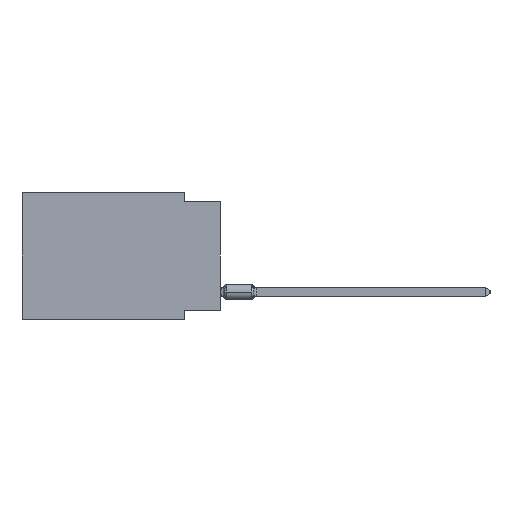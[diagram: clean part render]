
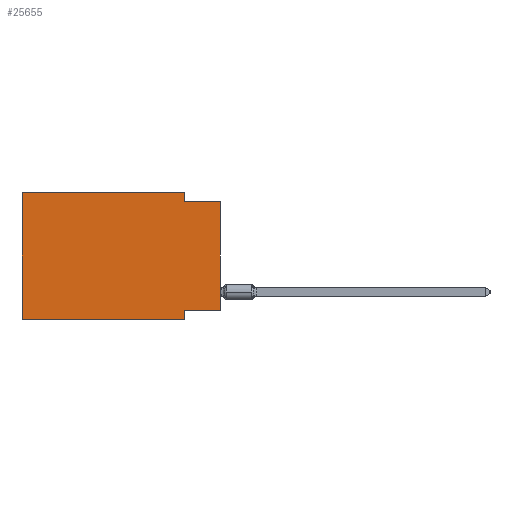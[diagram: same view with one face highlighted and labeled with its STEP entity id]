
A CAD part, left-side view. The second image highlights one B-rep face of the part: STEP entity #25655.
In plain terms, the highlighted planar face has unit normal (-1, 0, 0).
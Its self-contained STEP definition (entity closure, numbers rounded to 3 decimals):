
#2280 = VECTOR ( 'NONE', #48799, 1000. ) ;
#2856 = DIRECTION ( 'NONE',  ( 0., 1., 0. ) ) ;
#3340 = LINE ( 'NONE', #44732, #25423 ) ;
#3586 = CARTESIAN_POINT ( 'NONE',  ( 0., 13.97, 0. ) ) ;
#4630 = EDGE_LOOP ( 'NONE', ( #45822, #41184, #35078, #54529, #61562, #39311, #8893, #6857 ) ) ;
#4835 = EDGE_CURVE ( 'NONE', #22726, #38646, #18405, .T. ) ;
#6857 = ORIENTED_EDGE ( 'NONE', *, *, #37239, .F. ) ;
#8236 = CARTESIAN_POINT ( 'NONE',  ( 0., 2.54, -8.89 ) ) ;
#8479 = VECTOR ( 'NONE', #18309, 1000. ) ;
#8893 = ORIENTED_EDGE ( 'NONE', *, *, #59801, .F. ) ;
#9048 = PLANE ( 'NONE',  #47909 ) ;
#10798 = LINE ( 'NONE', #46864, #11913 ) ;
#11913 = VECTOR ( 'NONE', #29905, 1000. ) ;
#12756 = VERTEX_POINT ( 'NONE', #59773 ) ;
#14596 = CARTESIAN_POINT ( 'NONE',  ( 0., 2.54, 0. ) ) ;
#17453 = CARTESIAN_POINT ( 'NONE',  ( 0., 13.97, 0. ) ) ;
#18309 = DIRECTION ( 'NONE',  ( 0., -1., 0. ) ) ;
#18405 = LINE ( 'NONE', #28412, #2280 ) ;
#18553 = CARTESIAN_POINT ( 'NONE',  ( 0., 13.97, -8.89 ) ) ;
#19028 = VERTEX_POINT ( 'NONE', #32511 ) ;
#19071 = VERTEX_POINT ( 'NONE', #37526 ) ;
#19079 = DIRECTION ( 'NONE',  ( 1., 0., 0. ) ) ;
#19621 = LINE ( 'NONE', #28971, #8479 ) ;
#22726 = VERTEX_POINT ( 'NONE', #17453 ) ;
#24080 = VERTEX_POINT ( 'NONE', #52209 ) ;
#24137 = CARTESIAN_POINT ( 'NONE',  ( 0., 2.54, -8.255 ) ) ;
#24766 = VERTEX_POINT ( 'NONE', #59408 ) ;
#25423 = VECTOR ( 'NONE', #39058, 1000. ) ;
#25655 = ADVANCED_FACE ( 'NONE', ( #39110 ), #9048, .F. ) ;
#28234 = LINE ( 'NONE', #48616, #57501 ) ;
#28412 = CARTESIAN_POINT ( 'NONE',  ( 0., 13.97, 0. ) ) ;
#28971 = CARTESIAN_POINT ( 'NONE',  ( 0., 0., -0.635 ) ) ;
#29158 = EDGE_CURVE ( 'NONE', #19028, #24080, #10798, .T. ) ;
#29258 = DIRECTION ( 'NONE',  ( 0., 0., -1. ) ) ;
#29408 = CARTESIAN_POINT ( 'NONE',  ( 0., 13.97, 0. ) ) ;
#29905 = DIRECTION ( 'NONE',  ( 0., 0., 1. ) ) ;
#32064 = VERTEX_POINT ( 'NONE', #24137 ) ;
#32511 = CARTESIAN_POINT ( 'NONE',  ( 0., 0., -8.255 ) ) ;
#34122 = DIRECTION ( 'NONE',  ( 0., 0., -1. ) ) ;
#35078 = ORIENTED_EDGE ( 'NONE', *, *, #47516, .F. ) ;
#37239 = EDGE_CURVE ( 'NONE', #19028, #32064, #28234, .T. ) ;
#37526 = CARTESIAN_POINT ( 'NONE',  ( 0., 13.97, -8.89 ) ) ;
#38620 = EDGE_CURVE ( 'NONE', #24766, #24080, #19621, .T. ) ;
#38646 = VERTEX_POINT ( 'NONE', #14596 ) ;
#38920 = EDGE_CURVE ( 'NONE', #19071, #12756, #54632, .T. ) ;
#39058 = DIRECTION ( 'NONE',  ( 0., 0., -1. ) ) ;
#39110 = FACE_OUTER_BOUND ( 'NONE', #4630, .T. ) ;
#39311 = ORIENTED_EDGE ( 'NONE', *, *, #38920, .T. ) ;
#39898 = DIRECTION ( 'NONE',  ( 0., -1., 0. ) ) ;
#41184 = ORIENTED_EDGE ( 'NONE', *, *, #38620, .F. ) ;
#44732 = CARTESIAN_POINT ( 'NONE',  ( 0., 2.54, 0. ) ) ;
#45822 = ORIENTED_EDGE ( 'NONE', *, *, #29158, .T. ) ;
#46844 = VECTOR ( 'NONE', #29258, 1000. ) ;
#46864 = CARTESIAN_POINT ( 'NONE',  ( 0., 0., 0. ) ) ;
#47516 = EDGE_CURVE ( 'NONE', #38646, #24766, #3340, .T. ) ;
#47909 = AXIS2_PLACEMENT_3D ( 'NONE', #29408, #19079, #34122 ) ;
#48104 = VECTOR ( 'NONE', #50328, 1000. ) ;
#48616 = CARTESIAN_POINT ( 'NONE',  ( 0., 0., -8.255 ) ) ;
#48799 = DIRECTION ( 'NONE',  ( 0., -1., 0. ) ) ;
#49345 = LINE ( 'NONE', #3586, #48104 ) ;
#50328 = DIRECTION ( 'NONE',  ( 0., 0., 1. ) ) ;
#52209 = CARTESIAN_POINT ( 'NONE',  ( 0., 0., -0.635 ) ) ;
#54369 = VECTOR ( 'NONE', #39898, 1000. ) ;
#54529 = ORIENTED_EDGE ( 'NONE', *, *, #4835, .F. ) ;
#54632 = LINE ( 'NONE', #18553, #54369 ) ;
#56445 = EDGE_CURVE ( 'NONE', #19071, #22726, #49345, .T. ) ;
#57501 = VECTOR ( 'NONE', #2856, 1000. ) ;
#59408 = CARTESIAN_POINT ( 'NONE',  ( 0., 2.54, -0.635 ) ) ;
#59773 = CARTESIAN_POINT ( 'NONE',  ( 0., 2.54, -8.89 ) ) ;
#59801 = EDGE_CURVE ( 'NONE', #32064, #12756, #64361, .T. ) ;
#61562 = ORIENTED_EDGE ( 'NONE', *, *, #56445, .F. ) ;
#64361 = LINE ( 'NONE', #8236, #46844 ) ;
